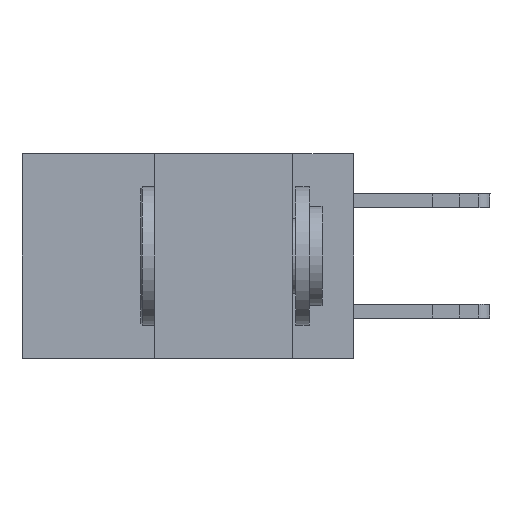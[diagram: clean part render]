
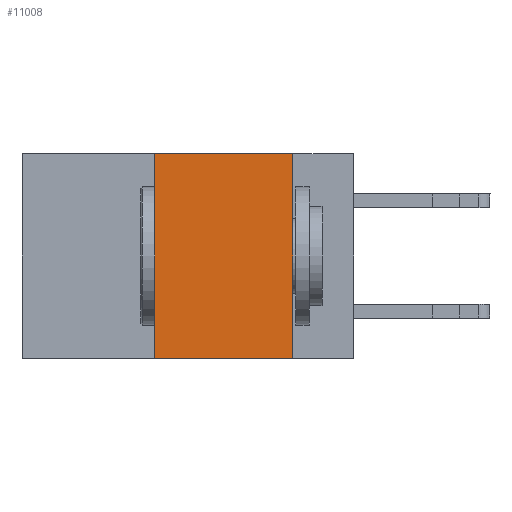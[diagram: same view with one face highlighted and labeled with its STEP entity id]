
A CAD part, left-side view. The second image highlights one B-rep face of the part: STEP entity #11008.
In plain terms, the highlighted planar face has unit normal (-1, 0, 0).
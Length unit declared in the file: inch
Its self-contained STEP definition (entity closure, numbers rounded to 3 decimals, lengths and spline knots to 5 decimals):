
#1610 = CARTESIAN_POINT ( 'NONE',  ( 0., 0.6, -0.37 ) ) ;
#2209 = DIRECTION ( 'NONE',  ( 0., 0., -1. ) ) ;
#2908 = DIRECTION ( 'NONE',  ( 0., -1., 0. ) ) ;
#3095 = CARTESIAN_POINT ( 'NONE',  ( 0., 0.11, -0.37 ) ) ;
#3321 = AXIS2_PLACEMENT_3D ( 'NONE', #5742, #15579, #8230 ) ;
#4161 = VERTEX_POINT ( 'NONE', #3095 ) ;
#4601 = CARTESIAN_POINT ( 'NONE',  ( 0., 0.6, 0. ) ) ;
#5113 = LINE ( 'NONE', #4601, #14173 ) ;
#5245 = DIRECTION ( 'NONE',  ( 0., 0., 1. ) ) ;
#5563 = CARTESIAN_POINT ( 'NONE',  ( 0., 0.36, 0. ) ) ;
#5742 = CARTESIAN_POINT ( 'NONE',  ( 0., 0.6, 0. ) ) ;
#6606 = VECTOR ( 'NONE', #5245, 39.37008 ) ;
#6721 = VECTOR ( 'NONE', #2908, 39.37008 ) ;
#6779 = VERTEX_POINT ( 'NONE', #11091 ) ;
#6992 = LINE ( 'NONE', #11384, #6606 ) ;
#7102 = LINE ( 'NONE', #1610, #6721 ) ;
#7177 = ORIENTED_EDGE ( 'NONE', *, *, #14320, .F. ) ;
#8159 = EDGE_CURVE ( 'NONE', #12685, #15556, #6992, .T. ) ;
#8230 = DIRECTION ( 'NONE',  ( 0., 0., -1. ) ) ;
#9686 = ORIENTED_EDGE ( 'NONE', *, *, #12474, .F. ) ;
#9688 = CARTESIAN_POINT ( 'NONE',  ( 0., 0.11, 0. ) ) ;
#10118 = CARTESIAN_POINT ( 'NONE',  ( 0., 0.36, -0.37 ) ) ;
#11008 = ADVANCED_FACE ( 'NONE', ( #11372 ), #14341, .F. ) ;
#11091 = CARTESIAN_POINT ( 'NONE',  ( 0., 0.11, 0. ) ) ;
#11372 = FACE_OUTER_BOUND ( 'NONE', #16112, .T. ) ;
#11384 = CARTESIAN_POINT ( 'NONE',  ( 0., 0.36, 0. ) ) ;
#11831 = ORIENTED_EDGE ( 'NONE', *, *, #12189, .T. ) ;
#11920 = LINE ( 'NONE', #9688, #15148 ) ;
#12002 = DIRECTION ( 'NONE',  ( 0., -1., 0. ) ) ;
#12189 = EDGE_CURVE ( 'NONE', #12685, #4161, #7102, .T. ) ;
#12474 = EDGE_CURVE ( 'NONE', #6779, #4161, #11920, .T. ) ;
#12685 = VERTEX_POINT ( 'NONE', #10118 ) ;
#14109 = ORIENTED_EDGE ( 'NONE', *, *, #8159, .F. ) ;
#14173 = VECTOR ( 'NONE', #12002, 39.37008 ) ;
#14320 = EDGE_CURVE ( 'NONE', #15556, #6779, #5113, .T. ) ;
#14341 = PLANE ( 'NONE',  #3321 ) ;
#15148 = VECTOR ( 'NONE', #2209, 39.37008 ) ;
#15556 = VERTEX_POINT ( 'NONE', #5563 ) ;
#15579 = DIRECTION ( 'NONE',  ( 1., 0., 0. ) ) ;
#16112 = EDGE_LOOP ( 'NONE', ( #9686, #7177, #14109, #11831 ) ) ;
